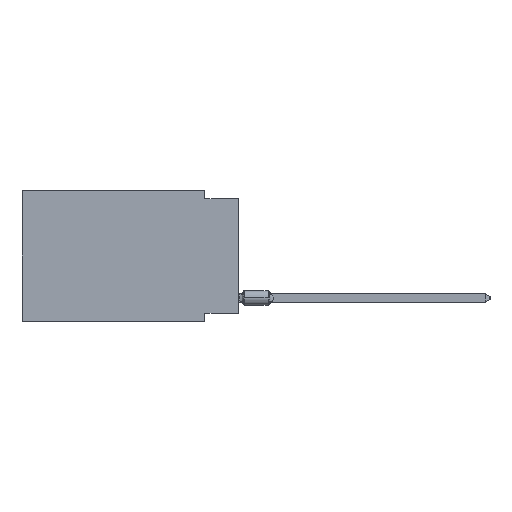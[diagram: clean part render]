
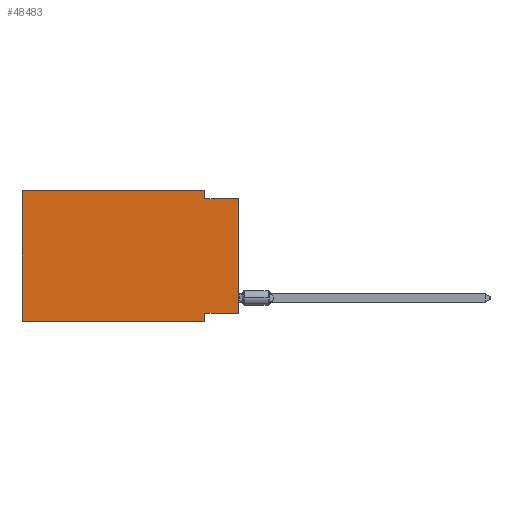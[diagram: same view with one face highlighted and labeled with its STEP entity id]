
A CAD part, left-side view. The second image highlights one B-rep face of the part: STEP entity #48483.
In plain terms, the highlighted planar face has unit normal (-1, 0, 0).
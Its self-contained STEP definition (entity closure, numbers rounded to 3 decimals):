
#1304 = CARTESIAN_POINT ( 'NONE',  ( 0., 16.383, 0. ) ) ;
#2593 = FACE_OUTER_BOUND ( 'NONE', #11824, .T. ) ;
#2693 = VERTEX_POINT ( 'NONE', #40483 ) ;
#3354 = VECTOR ( 'NONE', #25557, 1000. ) ;
#8246 = DIRECTION ( 'NONE',  ( 0., -1., 0. ) ) ;
#8425 = VERTEX_POINT ( 'NONE', #26881 ) ;
#10205 = CARTESIAN_POINT ( 'NONE',  ( 0., 2.54, -9.906 ) ) ;
#10434 = ORIENTED_EDGE ( 'NONE', *, *, #17764, .F. ) ;
#11416 = EDGE_CURVE ( 'NONE', #12088, #17989, #25268, .T. ) ;
#11824 = EDGE_LOOP ( 'NONE', ( #35467, #10434, #38377, #28610, #20083, #48062, #43724, #32345 ) ) ;
#12088 = VERTEX_POINT ( 'NONE', #36156 ) ;
#13181 = EDGE_CURVE ( 'NONE', #8425, #14821, #21807, .T. ) ;
#13527 = CARTESIAN_POINT ( 'NONE',  ( 0., 16.383, 0. ) ) ;
#13950 = CARTESIAN_POINT ( 'NONE',  ( 0., 2.54, 0. ) ) ;
#14116 = LINE ( 'NONE', #29450, #27833 ) ;
#14161 = CARTESIAN_POINT ( 'NONE',  ( 0., 16.383, 0. ) ) ;
#14821 = VERTEX_POINT ( 'NONE', #18960 ) ;
#14841 = CARTESIAN_POINT ( 'NONE',  ( 0., 0., -9.271 ) ) ;
#15854 = EDGE_CURVE ( 'NONE', #20604, #42976, #36403, .T. ) ;
#17232 = EDGE_CURVE ( 'NONE', #18561, #2693, #46669, .T. ) ;
#17764 = EDGE_CURVE ( 'NONE', #17989, #2693, #14116, .T. ) ;
#17952 = PLANE ( 'NONE',  #31458 ) ;
#17989 = VERTEX_POINT ( 'NONE', #20065 ) ;
#18561 = VERTEX_POINT ( 'NONE', #40593 ) ;
#18960 = CARTESIAN_POINT ( 'NONE',  ( 0., 2.54, -9.906 ) ) ;
#19807 = CARTESIAN_POINT ( 'NONE',  ( 0., 16.383, -9.906 ) ) ;
#20034 = DIRECTION ( 'NONE',  ( 0., -1., 0. ) ) ;
#20065 = CARTESIAN_POINT ( 'NONE',  ( 0., 2.54, -0.635 ) ) ;
#20083 = ORIENTED_EDGE ( 'NONE', *, *, #15854, .F. ) ;
#20284 = LINE ( 'NONE', #24301, #32742 ) ;
#20604 = VERTEX_POINT ( 'NONE', #19807 ) ;
#21369 = VECTOR ( 'NONE', #25029, 1000. ) ;
#21807 = LINE ( 'NONE', #10205, #3354 ) ;
#24301 = CARTESIAN_POINT ( 'NONE',  ( 0., 16.383, -9.906 ) ) ;
#25029 = DIRECTION ( 'NONE',  ( 0., 0., -1. ) ) ;
#25268 = LINE ( 'NONE', #13950, #21369 ) ;
#25557 = DIRECTION ( 'NONE',  ( 0., 0., -1. ) ) ;
#25732 = DIRECTION ( 'NONE',  ( 0., 0., -1. ) ) ;
#25981 = VECTOR ( 'NONE', #29346, 1000. ) ;
#26881 = CARTESIAN_POINT ( 'NONE',  ( 0., 2.54, -9.271 ) ) ;
#27279 = CARTESIAN_POINT ( 'NONE',  ( 0., 0., 0. ) ) ;
#27716 = LINE ( 'NONE', #1304, #28666 ) ;
#27833 = VECTOR ( 'NONE', #8246, 1000. ) ;
#28610 = ORIENTED_EDGE ( 'NONE', *, *, #30779, .F. ) ;
#28666 = VECTOR ( 'NONE', #46367, 1000. ) ;
#29346 = DIRECTION ( 'NONE',  ( 0., 0., 1. ) ) ;
#29450 = CARTESIAN_POINT ( 'NONE',  ( 0., 0., -0.635 ) ) ;
#29493 = DIRECTION ( 'NONE',  ( 1., 0., 0. ) ) ;
#30779 = EDGE_CURVE ( 'NONE', #42976, #12088, #27716, .T. ) ;
#31458 = AXIS2_PLACEMENT_3D ( 'NONE', #14161, #29493, #25732 ) ;
#32345 = ORIENTED_EDGE ( 'NONE', *, *, #44527, .F. ) ;
#32742 = VECTOR ( 'NONE', #20034, 1000. ) ;
#32989 = VECTOR ( 'NONE', #42481, 1000. ) ;
#34196 = LINE ( 'NONE', #14841, #32989 ) ;
#35467 = ORIENTED_EDGE ( 'NONE', *, *, #17232, .T. ) ;
#36156 = CARTESIAN_POINT ( 'NONE',  ( 0., 2.54, 0. ) ) ;
#36403 = LINE ( 'NONE', #44462, #25981 ) ;
#38377 = ORIENTED_EDGE ( 'NONE', *, *, #11416, .F. ) ;
#40483 = CARTESIAN_POINT ( 'NONE',  ( 0., 0., -0.635 ) ) ;
#40593 = CARTESIAN_POINT ( 'NONE',  ( 0., 0., -9.271 ) ) ;
#40683 = EDGE_CURVE ( 'NONE', #20604, #14821, #20284, .T. ) ;
#42481 = DIRECTION ( 'NONE',  ( 0., 1., 0. ) ) ;
#42976 = VERTEX_POINT ( 'NONE', #13527 ) ;
#43724 = ORIENTED_EDGE ( 'NONE', *, *, #13181, .F. ) ;
#44462 = CARTESIAN_POINT ( 'NONE',  ( 0., 16.383, 0. ) ) ;
#44527 = EDGE_CURVE ( 'NONE', #18561, #8425, #34196, .T. ) ;
#46367 = DIRECTION ( 'NONE',  ( 0., -1., 0. ) ) ;
#46669 = LINE ( 'NONE', #27279, #48707 ) ;
#46923 = DIRECTION ( 'NONE',  ( 0., 0., 1. ) ) ;
#48062 = ORIENTED_EDGE ( 'NONE', *, *, #40683, .T. ) ;
#48483 = ADVANCED_FACE ( 'NONE', ( #2593 ), #17952, .F. ) ;
#48707 = VECTOR ( 'NONE', #46923, 1000. ) ;
